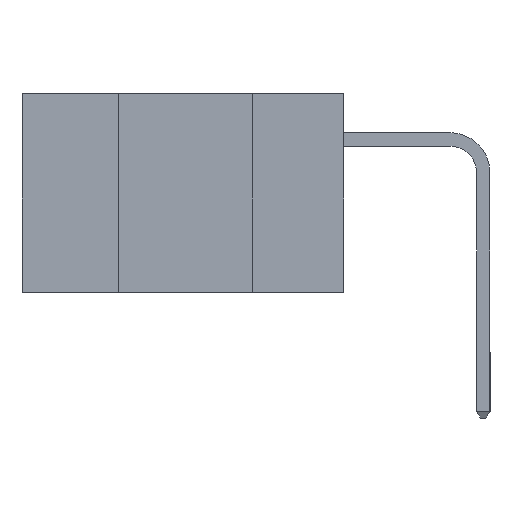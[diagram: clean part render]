
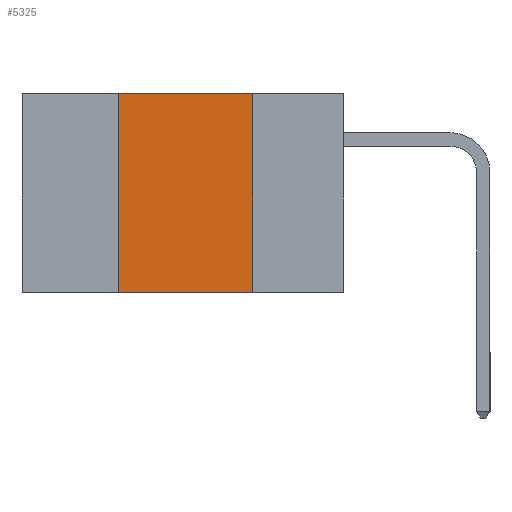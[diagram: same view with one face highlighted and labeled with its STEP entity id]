
A CAD part, left-side view. The second image highlights one B-rep face of the part: STEP entity #5325.
In plain terms, the highlighted planar face has unit normal (-1, 0, 0).
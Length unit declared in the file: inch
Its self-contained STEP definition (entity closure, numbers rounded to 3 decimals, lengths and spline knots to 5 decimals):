
#327 = VERTEX_POINT ( 'NONE', #6653 ) ;
#2565 = VECTOR ( 'NONE', #9101, 39.37008 ) ;
#2942 = ORIENTED_EDGE ( 'NONE', *, *, #3828, .F. ) ;
#2989 = CARTESIAN_POINT ( 'NONE',  ( 0., 0.6, 0. ) ) ;
#3334 = VERTEX_POINT ( 'NONE', #4736 ) ;
#3401 = DIRECTION ( 'NONE',  ( 0., -1., 0. ) ) ;
#3719 = ORIENTED_EDGE ( 'NONE', *, *, #9766, .T. ) ;
#3828 = EDGE_CURVE ( 'NONE', #14117, #4618, #9067, .T. ) ;
#4169 = CARTESIAN_POINT ( 'NONE',  ( 0., 0.17, 0. ) ) ;
#4618 = VERTEX_POINT ( 'NONE', #4738 ) ;
#4736 = CARTESIAN_POINT ( 'NONE',  ( 0., 0.42, 0. ) ) ;
#4738 = CARTESIAN_POINT ( 'NONE',  ( 0., 0.17, -0.37 ) ) ;
#4861 = ORIENTED_EDGE ( 'NONE', *, *, #11472, .F. ) ;
#5325 = ADVANCED_FACE ( 'NONE', ( #8763 ), #13465, .F. ) ;
#5735 = LINE ( 'NONE', #11550, #2565 ) ;
#6107 = ORIENTED_EDGE ( 'NONE', *, *, #9074, .F. ) ;
#6499 = DIRECTION ( 'NONE',  ( 1., 0., 0. ) ) ;
#6653 = CARTESIAN_POINT ( 'NONE',  ( 0., 0.42, -0.37 ) ) ;
#7387 = CARTESIAN_POINT ( 'NONE',  ( 0., 0.6, 0. ) ) ;
#7850 = VECTOR ( 'NONE', #14281, 39.37008 ) ;
#8763 = FACE_OUTER_BOUND ( 'NONE', #12789, .T. ) ;
#9067 = LINE ( 'NONE', #10303, #14818 ) ;
#9074 = EDGE_CURVE ( 'NONE', #3334, #14117, #9854, .T. ) ;
#9101 = DIRECTION ( 'NONE',  ( 0., 0., 1. ) ) ;
#9271 = LINE ( 'NONE', #11640, #11820 ) ;
#9766 = EDGE_CURVE ( 'NONE', #327, #4618, #9271, .T. ) ;
#9854 = LINE ( 'NONE', #7387, #7850 ) ;
#10303 = CARTESIAN_POINT ( 'NONE',  ( 0., 0.17, -0.37 ) ) ;
#11174 = DIRECTION ( 'NONE',  ( 0., 0., -1. ) ) ;
#11472 = EDGE_CURVE ( 'NONE', #327, #3334, #5735, .T. ) ;
#11550 = CARTESIAN_POINT ( 'NONE',  ( 0., 0.42, -0.37 ) ) ;
#11640 = CARTESIAN_POINT ( 'NONE',  ( 0., 0.6, -0.37 ) ) ;
#11820 = VECTOR ( 'NONE', #3401, 39.37008 ) ;
#12599 = DIRECTION ( 'NONE',  ( 0., 0., -1. ) ) ;
#12789 = EDGE_LOOP ( 'NONE', ( #2942, #6107, #4861, #3719 ) ) ;
#13185 = AXIS2_PLACEMENT_3D ( 'NONE', #2989, #6499, #11174 ) ;
#13465 = PLANE ( 'NONE',  #13185 ) ;
#14117 = VERTEX_POINT ( 'NONE', #4169 ) ;
#14281 = DIRECTION ( 'NONE',  ( 0., -1., 0. ) ) ;
#14818 = VECTOR ( 'NONE', #12599, 39.37008 ) ;
